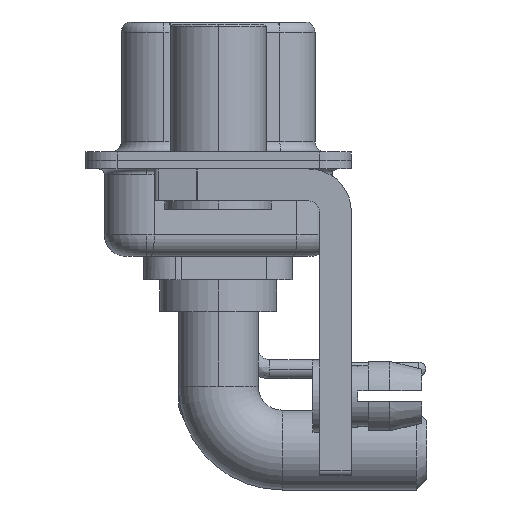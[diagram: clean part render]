
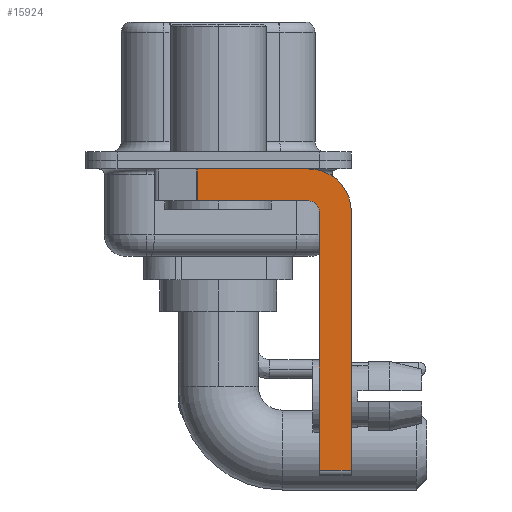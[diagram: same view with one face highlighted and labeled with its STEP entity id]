
A CAD part, left-side view. The second image highlights one B-rep face of the part: STEP entity #15924.
In plain terms, the highlighted planar face has unit normal (-1, 0, 0).
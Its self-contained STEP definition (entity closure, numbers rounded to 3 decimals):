
#316 = EDGE_LOOP ( 'NONE', ( #10574, #8991, #28855, #18306, #2974, #18578, #22833, #28888 ) ) ;
#1273 = VERTEX_POINT ( 'NONE', #23353 ) ;
#1519 = EDGE_CURVE ( 'NONE', #1273, #3022, #20153, .T. ) ;
#2187 = LINE ( 'NONE', #4433, #4749 ) ;
#2479 = CARTESIAN_POINT ( 'NONE',  ( -2.9, -6.25, -2.4 ) ) ;
#2480 = CARTESIAN_POINT ( 'NONE',  ( -2.9, -4.25, -1.9 ) ) ;
#2748 = VERTEX_POINT ( 'NONE', #2479 ) ;
#2974 = ORIENTED_EDGE ( 'NONE', *, *, #6574, .F. ) ;
#3022 = VERTEX_POINT ( 'NONE', #11627 ) ;
#3620 = LINE ( 'NONE', #12694, #12160 ) ;
#3928 = CARTESIAN_POINT ( 'NONE',  ( -2.9, -4.25, -2.4 ) ) ;
#4262 = DIRECTION ( 'NONE',  ( 0., 0., -1. ) ) ;
#4351 = CARTESIAN_POINT ( 'NONE',  ( -2.9, -4.75, -14.55 ) ) ;
#4427 = EDGE_CURVE ( 'NONE', #3022, #2748, #9657, .T. ) ;
#4433 = CARTESIAN_POINT ( 'NONE',  ( -2.9, 0.978, -1.9 ) ) ;
#4749 = VECTOR ( 'NONE', #9120, 1000. ) ;
#5630 = VERTEX_POINT ( 'NONE', #2480 ) ;
#6048 = DIRECTION ( 'NONE',  ( 0., 1., 0. ) ) ;
#6346 = PLANE ( 'NONE',  #10371 ) ;
#6574 = EDGE_CURVE ( 'NONE', #12657, #13396, #18483, .T. ) ;
#7034 = EDGE_CURVE ( 'NONE', #1273, #14208, #2187, .T. ) ;
#7187 = VERTEX_POINT ( 'NONE', #28243 ) ;
#7632 = DIRECTION ( 'NONE',  ( 0., 0., 1. ) ) ;
#8696 = VECTOR ( 'NONE', #17180, 1000. ) ;
#8759 = DIRECTION ( 'NONE',  ( 0., 0., -1. ) ) ;
#8991 = ORIENTED_EDGE ( 'NONE', *, *, #7034, .T. ) ;
#9120 = DIRECTION ( 'NONE',  ( 0., 0., -1. ) ) ;
#9629 = EDGE_CURVE ( 'NONE', #12657, #7187, #19884, .T. ) ;
#9657 = CIRCLE ( 'NONE', #28905, 2. ) ;
#9876 = CARTESIAN_POINT ( 'NONE',  ( -2.9, -4.75, -2.4 ) ) ;
#10371 = AXIS2_PLACEMENT_3D ( 'NONE', #3928, #13143, #8759 ) ;
#10574 = ORIENTED_EDGE ( 'NONE', *, *, #1519, .F. ) ;
#11328 = FACE_OUTER_BOUND ( 'NONE', #316, .T. ) ;
#11627 = CARTESIAN_POINT ( 'NONE',  ( -2.9, -4.25, -0.4 ) ) ;
#12160 = VECTOR ( 'NONE', #6048, 1000. ) ;
#12432 = CARTESIAN_POINT ( 'NONE',  ( -2.9, -4.25, -2.4 ) ) ;
#12657 = VERTEX_POINT ( 'NONE', #4351 ) ;
#12694 = CARTESIAN_POINT ( 'NONE',  ( -2.9, -4.25, -1.9 ) ) ;
#13143 = DIRECTION ( 'NONE',  ( 1., 0., 0. ) ) ;
#13221 = DIRECTION ( 'NONE',  ( -1., 0., 0. ) ) ;
#13396 = VERTEX_POINT ( 'NONE', #9876 ) ;
#13630 = VECTOR ( 'NONE', #7632, 1000. ) ;
#14208 = VERTEX_POINT ( 'NONE', #23078 ) ;
#14915 = CARTESIAN_POINT ( 'NONE',  ( -2.9, -4.25, -14.55 ) ) ;
#15783 = CARTESIAN_POINT ( 'NONE',  ( -2.9, -4.25, -2.4 ) ) ;
#15924 = ADVANCED_FACE ( 'NONE', ( #11328 ), #6346, .F. ) ;
#15931 = DIRECTION ( 'NONE',  ( 0., 0., 1. ) ) ;
#16221 = CARTESIAN_POINT ( 'NONE',  ( -2.9, -4.75, -14.8 ) ) ;
#17180 = DIRECTION ( 'NONE',  ( 0., -1., 0. ) ) ;
#17698 = VECTOR ( 'NONE', #27068, 1000. ) ;
#18127 = EDGE_CURVE ( 'NONE', #13396, #5630, #22538, .T. ) ;
#18306 = ORIENTED_EDGE ( 'NONE', *, *, #18127, .F. ) ;
#18337 = VECTOR ( 'NONE', #4262, 1000. ) ;
#18483 = LINE ( 'NONE', #16221, #13630 ) ;
#18578 = ORIENTED_EDGE ( 'NONE', *, *, #9629, .T. ) ;
#19884 = LINE ( 'NONE', #14915, #8696 ) ;
#20002 = CARTESIAN_POINT ( 'NONE',  ( -2.9, 3., -0.4 ) ) ;
#20153 = LINE ( 'NONE', #20002, #17698 ) ;
#21348 = EDGE_CURVE ( 'NONE', #2748, #7187, #22539, .T. ) ;
#21632 = DIRECTION ( 'NONE',  ( 1., 0., 0. ) ) ;
#21710 = EDGE_CURVE ( 'NONE', #5630, #14208, #3620, .T. ) ;
#22056 = AXIS2_PLACEMENT_3D ( 'NONE', #15783, #13221, #15931 ) ;
#22538 = CIRCLE ( 'NONE', #22056, 0.5 ) ;
#22539 = LINE ( 'NONE', #24928, #18337 ) ;
#22833 = ORIENTED_EDGE ( 'NONE', *, *, #21348, .F. ) ;
#23078 = CARTESIAN_POINT ( 'NONE',  ( -2.9, 0.978, -1.9 ) ) ;
#23353 = CARTESIAN_POINT ( 'NONE',  ( -2.9, 0.978, -0.4 ) ) ;
#24928 = CARTESIAN_POINT ( 'NONE',  ( -2.9, -6.25, -2.4 ) ) ;
#27068 = DIRECTION ( 'NONE',  ( 0., -1., 0. ) ) ;
#28093 = DIRECTION ( 'NONE',  ( 0., 0., -1. ) ) ;
#28243 = CARTESIAN_POINT ( 'NONE',  ( -2.9, -6.25, -14.55 ) ) ;
#28855 = ORIENTED_EDGE ( 'NONE', *, *, #21710, .F. ) ;
#28888 = ORIENTED_EDGE ( 'NONE', *, *, #4427, .F. ) ;
#28905 = AXIS2_PLACEMENT_3D ( 'NONE', #12432, #21632, #28093 ) ;
